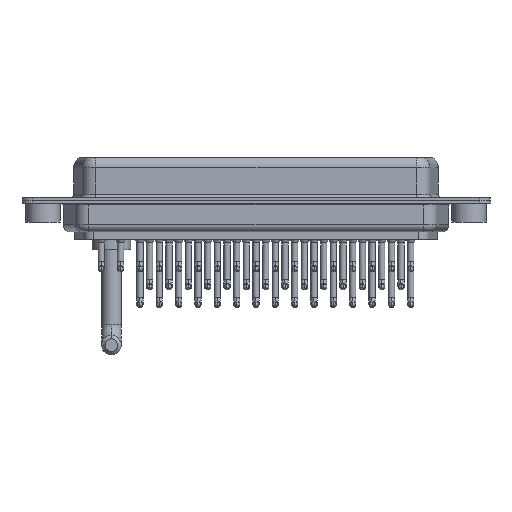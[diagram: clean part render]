
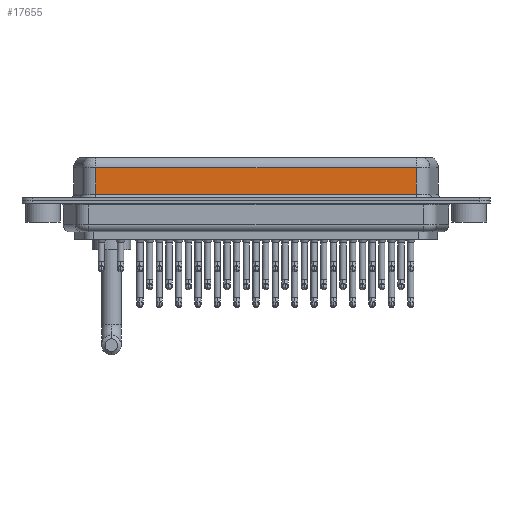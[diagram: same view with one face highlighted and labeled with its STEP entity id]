
A CAD part, front view. The second image highlights one B-rep face of the part: STEP entity #17655.
In plain terms, the highlighted planar face has unit normal (0, -1, 0).
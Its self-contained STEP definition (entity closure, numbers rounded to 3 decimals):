
#869 = LINE ( 'NONE', #19600, #30471 ) ;
#2613 = EDGE_CURVE ( 'NONE', #26171, #15381, #24652, .T. ) ;
#4312 = CARTESIAN_POINT ( 'NONE',  ( 7.59, -5.375, 0.9 ) ) ;
#4474 = FACE_OUTER_BOUND ( 'NONE', #28970, .T. ) ;
#5162 = AXIS2_PLACEMENT_3D ( 'NONE', #12369, #20283, #9961 ) ;
#9359 = EDGE_CURVE ( 'NONE', #23025, #26171, #869, .T. ) ;
#9648 = ORIENTED_EDGE ( 'NONE', *, *, #2613, .T. ) ;
#9956 = DIRECTION ( 'NONE',  ( -1., 0., 0. ) ) ;
#9961 = DIRECTION ( 'NONE',  ( 0., 0., 1. ) ) ;
#11687 = VECTOR ( 'NONE', #9956, 1000. ) ;
#11983 = ORIENTED_EDGE ( 'NONE', *, *, #32882, .F. ) ;
#12369 = CARTESIAN_POINT ( 'NONE',  ( 53.41, -5.375, 6.4 ) ) ;
#13804 = ORIENTED_EDGE ( 'NONE', *, *, #16343, .T. ) ;
#14059 = VERTEX_POINT ( 'NONE', #27088 ) ;
#14265 = VECTOR ( 'NONE', #26471, 1000. ) ;
#15381 = VERTEX_POINT ( 'NONE', #18742 ) ;
#15962 = CARTESIAN_POINT ( 'NONE',  ( 53.41, -5.375, 6.4 ) ) ;
#16343 = EDGE_CURVE ( 'NONE', #14059, #23025, #25113, .T. ) ;
#16673 = DIRECTION ( 'NONE',  ( 0., 0., -1. ) ) ;
#16740 = DIRECTION ( 'NONE',  ( 1., 0., 0. ) ) ;
#17655 = ADVANCED_FACE ( 'NONE', ( #4474 ), #25795, .F. ) ;
#18742 = CARTESIAN_POINT ( 'NONE',  ( 53.41, -5.375, 0.9 ) ) ;
#19600 = CARTESIAN_POINT ( 'NONE',  ( 7.59, -5.375, 6.4 ) ) ;
#20283 = DIRECTION ( 'NONE',  ( 0., 1., 0. ) ) ;
#21896 = CARTESIAN_POINT ( 'NONE',  ( 53.41, -5.375, 0.9 ) ) ;
#23025 = VERTEX_POINT ( 'NONE', #29382 ) ;
#24230 = LINE ( 'NONE', #15962, #14265 ) ;
#24652 = LINE ( 'NONE', #21896, #26279 ) ;
#25113 = LINE ( 'NONE', #28377, #11687 ) ;
#25795 = PLANE ( 'NONE',  #5162 ) ;
#26171 = VERTEX_POINT ( 'NONE', #4312 ) ;
#26279 = VECTOR ( 'NONE', #16740, 1000. ) ;
#26471 = DIRECTION ( 'NONE',  ( 0., 0., -1. ) ) ;
#27088 = CARTESIAN_POINT ( 'NONE',  ( 53.41, -5.375, 4.65 ) ) ;
#28377 = CARTESIAN_POINT ( 'NONE',  ( 53.41, -5.375, 4.65 ) ) ;
#28970 = EDGE_LOOP ( 'NONE', ( #11983, #13804, #29670, #9648 ) ) ;
#29382 = CARTESIAN_POINT ( 'NONE',  ( 7.59, -5.375, 4.65 ) ) ;
#29670 = ORIENTED_EDGE ( 'NONE', *, *, #9359, .T. ) ;
#30471 = VECTOR ( 'NONE', #16673, 1000. ) ;
#32882 = EDGE_CURVE ( 'NONE', #14059, #15381, #24230, .T. ) ;
